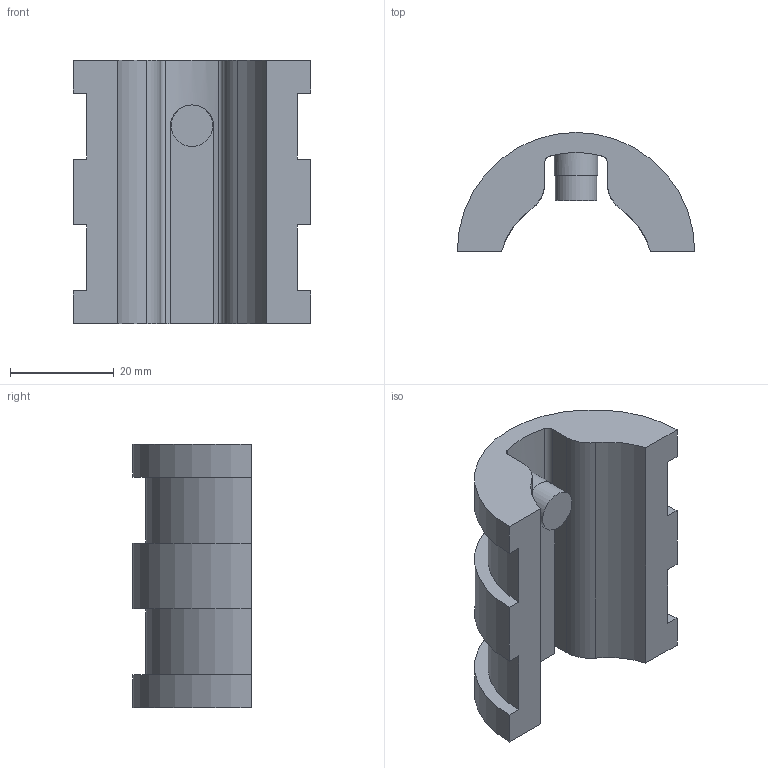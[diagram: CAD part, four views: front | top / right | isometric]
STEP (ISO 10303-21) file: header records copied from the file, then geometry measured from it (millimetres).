
FILE_DESCRIPTION (( 'STEP AP214' ), '1' );
FILE_NAME ('Trellais_Base_2.step', '2016-04-19T10:44:27', ( 'WarFairy' ), ( '' ), 'SwSTEP 2.0', 'SolidWorks 2015', '' );
FILE_SCHEMA (( 'AUTOMOTIVE_DESIGN' ));
Length unit declared in the file: inch
Products named in the file (1): Trellais_Base_2
Bounding box: 45.72 x 22.86 x 50.8 mm (x, y, z)
Volume: 22127.3 mm3; surface area: 9070.2 mm2
Topology: 1 solids, 1 shells, 28 faces, 77 edges, 51 vertices
Faces by surface type: plane 14, cylinder 14
Full cylindrical faces by diameter (mm): 8.001 x1
Entity records: 959 total; most frequent: CARTESIAN_POINT 187, DIRECTION 161, ORIENTED_EDGE 150, EDGE_CURVE 75, AXIS2_PLACEMENT_3D 58, VERTEX_POINT 50, LINE 45, VECTOR 45
